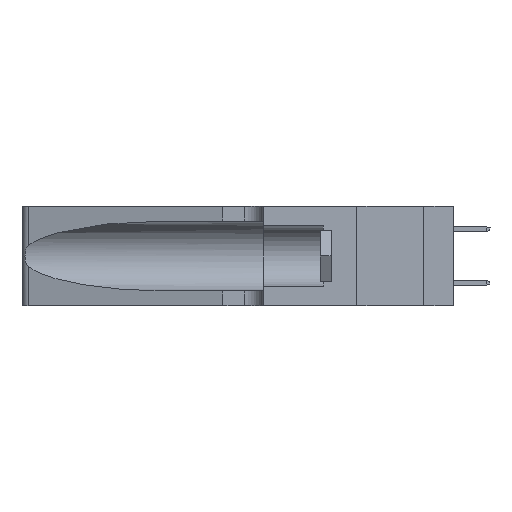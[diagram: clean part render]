
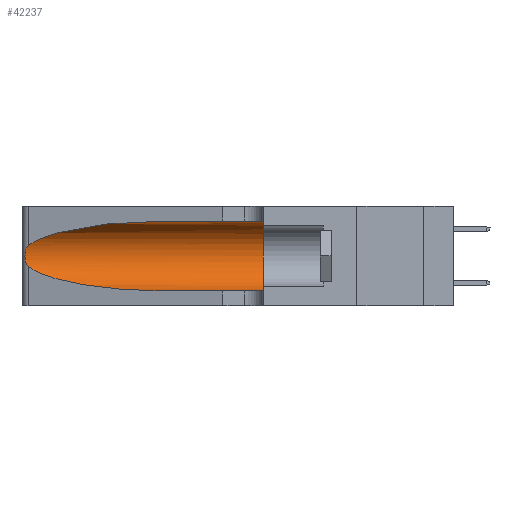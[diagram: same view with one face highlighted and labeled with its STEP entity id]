
A CAD part, left-side view. The second image highlights one B-rep face of the part: STEP entity #42237.
In plain terms, the highlighted cylindrical face has radius 3.308 mm (diameter 6.617 mm), a partial arc.
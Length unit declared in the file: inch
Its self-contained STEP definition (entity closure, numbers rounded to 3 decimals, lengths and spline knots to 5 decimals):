
#485 = VERTEX_POINT ( 'NONE', #19207 ) ;
#546 = CARTESIAN_POINT ( 'NONE',  ( 0.18966, 0.96281, 0.05475 ) ) ;
#740 = EDGE_LOOP ( 'NONE', ( #29495, #46601, #41646, #48552, #35278, #45097 ) ) ;
#1973 = VERTEX_POINT ( 'NONE', #34217 ) ;
#2404 = CARTESIAN_POINT ( 'NONE',  ( 0.1305, 1.61858, 0.31525 ) ) ;
#2408 =( BOUNDED_CURVE ( )  B_SPLINE_CURVE ( 3, ( #46403, #45676, #546, #26841 ),
 .UNSPECIFIED., .F., .T. ) 
 B_SPLINE_CURVE_WITH_KNOTS ( ( 4, 4 ),
 ( 3.44316, 4.71239 ),
 .UNSPECIFIED. ) 
 CURVE ( )  GEOMETRIC_REPRESENTATION_ITEM ( )  RATIONAL_B_SPLINE_CURVE ( ( 1., 0.87, 0.87, 1. ) ) 
 REPRESENTATION_ITEM ( '' )  );
#2966 = VECTOR ( 'NONE', #44313, 39.37008 ) ;
#3002 = CARTESIAN_POINT ( 'NONE',  ( 0.25487, 1.22718, 0.22369 ) ) ;
#3234 = CARTESIAN_POINT ( 'NONE',  ( 0.25487, 1.22718, 0.22369 ) ) ;
#3832 = VERTEX_POINT ( 'NONE', #4137 ) ;
#3959 = CARTESIAN_POINT ( 'NONE',  ( 0.2373, 1.15595, 0.28018 ) ) ;
#4137 = CARTESIAN_POINT ( 'NONE',  ( 0.1305, 0.72297, 0.31525 ) ) ;
#4384 = AXIS2_PLACEMENT_3D ( 'NONE', #43358, #6405, #17581 ) ;
#5106 = CARTESIAN_POINT ( 'NONE',  ( 0.25555, 1.22993, 0.14849 ) ) ;
#6405 = DIRECTION ( 'NONE',  ( 0., 1., 0. ) ) ;
#8220 = EDGE_CURVE ( 'NONE', #3832, #29749, #36308, .T. ) ;
#9475 = EDGE_CURVE ( 'NONE', #3832, #1973, #20334, .T. ) ;
#10690 = CARTESIAN_POINT ( 'NONE',  ( 0.25639, 1.23184, 0.21858 ) ) ;
#11413 = CARTESIAN_POINT ( 'NONE',  ( 0.1305, 0.72297, 0.05475 ) ) ;
#11842 = CARTESIAN_POINT ( 'NONE',  ( 0.25854, 1.2359, 0.20912 ) ) ;
#15815 = CARTESIAN_POINT ( 'NONE',  ( 0.26075, 1.23896, 0.178 ) ) ;
#17393 = EDGE_CURVE ( 'NONE', #23069, #485, #29674, .T. ) ;
#17581 = DIRECTION ( 'NONE',  ( 0., 0., 1. ) ) ;
#18768 = CARTESIAN_POINT ( 'NONE',  ( 0.1305, 1.61858, 0.05475 ) ) ;
#19207 = CARTESIAN_POINT ( 'NONE',  ( 0.1305, 0.35, 0.05475 ) ) ;
#20095 = VERTEX_POINT ( 'NONE', #39958 ) ;
#20334 = LINE ( 'NONE', #2404, #2966 ) ;
#22961 = B_SPLINE_CURVE_WITH_KNOTS ( 'NONE', 3,
 ( #3002, #48405, #10690, #25823, #11842, #46547, #46054, #15815, #23227, #27449, #23719, #31660, #5106, #23967 ),
 .UNSPECIFIED., .F., .F.,
 ( 4, 2, 2, 2, 2, 2, 4 ),
 ( 0., 0.00027, 0.00053, 0.00107, 0.0016, 0.00187, 0.00214 ),
 .UNSPECIFIED. ) ;
#23069 = VERTEX_POINT ( 'NONE', #11413 ) ;
#23155 = DIRECTION ( 'NONE',  ( 0., -1., 0. ) ) ;
#23227 = CARTESIAN_POINT ( 'NONE',  ( 0.26017, 1.23833, 0.17102 ) ) ;
#23719 = CARTESIAN_POINT ( 'NONE',  ( 0.25789, 1.23486, 0.15765 ) ) ;
#23967 = CARTESIAN_POINT ( 'NONE',  ( 0.25487, 1.22718, 0.14631 ) ) ;
#25823 = CARTESIAN_POINT ( 'NONE',  ( 0.25787, 1.23484, 0.2124 ) ) ;
#26841 = CARTESIAN_POINT ( 'NONE',  ( 0.1305, 0.72297, 0.05475 ) ) ;
#27134 = CARTESIAN_POINT ( 'NONE',  ( 0.1305, 1.61858, 0.185 ) ) ;
#27449 = CARTESIAN_POINT ( 'NONE',  ( 0.25856, 1.23593, 0.16098 ) ) ;
#27972 = EDGE_CURVE ( 'NONE', #20095, #23069, #2408, .T. ) ;
#29495 = ORIENTED_EDGE ( 'NONE', *, *, #8220, .T. ) ;
#29674 = LINE ( 'NONE', #18768, #44602 ) ;
#29749 = VERTEX_POINT ( 'NONE', #34725 ) ;
#30165 = DIRECTION ( 'NONE',  ( 0., -1., 0. ) ) ;
#31140 = AXIS2_PLACEMENT_3D ( 'NONE', #27134, #23155, #41523 ) ;
#31660 = CARTESIAN_POINT ( 'NONE',  ( 0.25639, 1.23186, 0.15144 ) ) ;
#33155 = EDGE_CURVE ( 'NONE', #1973, #485, #48789, .T. ) ;
#34217 = CARTESIAN_POINT ( 'NONE',  ( 0.1305, 0.35, 0.31525 ) ) ;
#34725 = CARTESIAN_POINT ( 'NONE',  ( 0.25487, 1.22718, 0.22369 ) ) ;
#35061 = FACE_OUTER_BOUND ( 'NONE', #740, .T. ) ;
#35278 = ORIENTED_EDGE ( 'NONE', *, *, #33155, .F. ) ;
#36308 =( BOUNDED_CURVE ( )  B_SPLINE_CURVE ( 3, ( #45132, #37949, #3959, #3234 ),
 .UNSPECIFIED., .F., .F. ) 
 B_SPLINE_CURVE_WITH_KNOTS ( ( 4, 4 ),
 ( 1.5708, 2.84003 ),
 .UNSPECIFIED. ) 
 CURVE ( )  GEOMETRIC_REPRESENTATION_ITEM ( )  RATIONAL_B_SPLINE_CURVE ( ( 1., 0.87, 0.87, 1. ) ) 
 REPRESENTATION_ITEM ( '' )  );
#37653 = EDGE_CURVE ( 'NONE', #29749, #20095, #22961, .T. ) ;
#37828 = CYLINDRICAL_SURFACE ( 'NONE', #31140, 0.13025 ) ;
#37949 = CARTESIAN_POINT ( 'NONE',  ( 0.18966, 0.96281, 0.31525 ) ) ;
#39958 = CARTESIAN_POINT ( 'NONE',  ( 0.25487, 1.22718, 0.14631 ) ) ;
#41523 = DIRECTION ( 'NONE',  ( 0., 0., -1. ) ) ;
#41646 = ORIENTED_EDGE ( 'NONE', *, *, #27972, .T. ) ;
#42237 = ADVANCED_FACE ( 'NONE', ( #35061 ), #37828, .F. ) ;
#43358 = CARTESIAN_POINT ( 'NONE',  ( 0.1305, 0.35, 0.185 ) ) ;
#44313 = DIRECTION ( 'NONE',  ( 0., -1., 0. ) ) ;
#44602 = VECTOR ( 'NONE', #30165, 39.37008 ) ;
#45097 = ORIENTED_EDGE ( 'NONE', *, *, #9475, .F. ) ;
#45132 = CARTESIAN_POINT ( 'NONE',  ( 0.1305, 0.72297, 0.31525 ) ) ;
#45676 = CARTESIAN_POINT ( 'NONE',  ( 0.2373, 1.15595, 0.08982 ) ) ;
#46054 = CARTESIAN_POINT ( 'NONE',  ( 0.26075, 1.23896, 0.19203 ) ) ;
#46403 = CARTESIAN_POINT ( 'NONE',  ( 0.25487, 1.22718, 0.14631 ) ) ;
#46547 = CARTESIAN_POINT ( 'NONE',  ( 0.26018, 1.23835, 0.19895 ) ) ;
#46601 = ORIENTED_EDGE ( 'NONE', *, *, #37653, .T. ) ;
#48405 = CARTESIAN_POINT ( 'NONE',  ( 0.25555, 1.22994, 0.2215 ) ) ;
#48552 = ORIENTED_EDGE ( 'NONE', *, *, #17393, .T. ) ;
#48789 = CIRCLE ( 'NONE', #4384, 0.13025 ) ;
